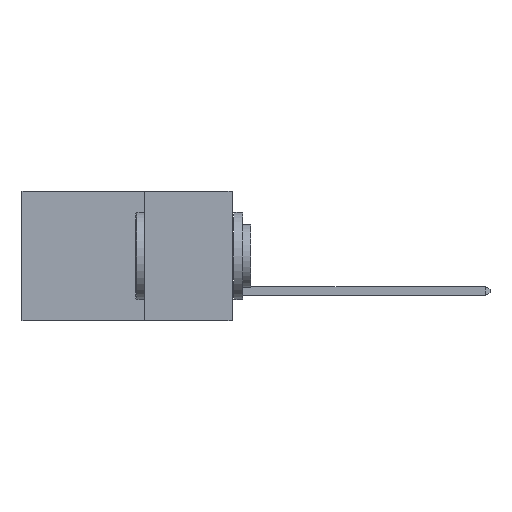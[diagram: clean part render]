
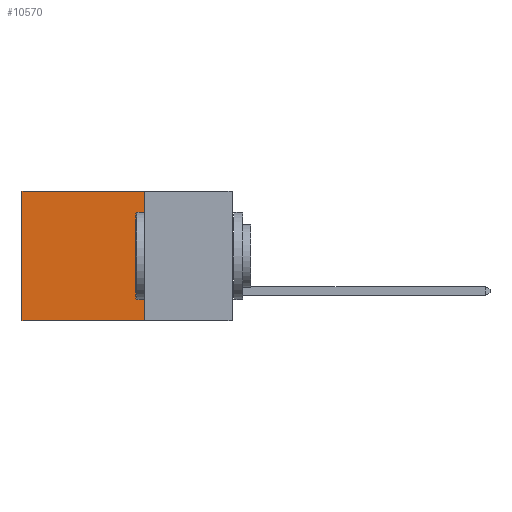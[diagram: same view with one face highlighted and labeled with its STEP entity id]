
A CAD part, left-side view. The second image highlights one B-rep face of the part: STEP entity #10570.
In plain terms, the highlighted planar face has unit normal (-1, 0, 0).
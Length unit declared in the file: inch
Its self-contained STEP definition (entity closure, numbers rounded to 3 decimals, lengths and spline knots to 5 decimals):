
#978 = VECTOR ( 'NONE', #19022, 39.37008 ) ;
#990 = VERTEX_POINT ( 'NONE', #17143 ) ;
#3026 = VECTOR ( 'NONE', #17542, 39.37008 ) ;
#3767 = DIRECTION ( 'NONE',  ( 1., 0., 0. ) ) ;
#4376 = LINE ( 'NONE', #12175, #12328 ) ;
#5429 = VERTEX_POINT ( 'NONE', #9429 ) ;
#5450 = LINE ( 'NONE', #17532, #978 ) ;
#7081 = VERTEX_POINT ( 'NONE', #13570 ) ;
#7306 = LINE ( 'NONE', #10642, #11495 ) ;
#7717 = VERTEX_POINT ( 'NONE', #15780 ) ;
#7954 = FACE_OUTER_BOUND ( 'NONE', #17458, .T. ) ;
#9429 = CARTESIAN_POINT ( 'NONE',  ( 0.2875, 0.6, 0. ) ) ;
#10570 = ADVANCED_FACE ( 'NONE', ( #7954 ), #13247, .F. ) ;
#10642 = CARTESIAN_POINT ( 'NONE',  ( 0.2875, 0.6, 0. ) ) ;
#10745 = EDGE_CURVE ( 'NONE', #990, #7081, #4376, .T. ) ;
#11495 = VECTOR ( 'NONE', #12145, 39.37008 ) ;
#12145 = DIRECTION ( 'NONE',  ( 0., 0., -1. ) ) ;
#12175 = CARTESIAN_POINT ( 'NONE',  ( 0.2875, 0.25, -0.37 ) ) ;
#12304 = AXIS2_PLACEMENT_3D ( 'NONE', #19139, #3767, #14733 ) ;
#12328 = VECTOR ( 'NONE', #13682, 39.37008 ) ;
#13247 = PLANE ( 'NONE',  #12304 ) ;
#13538 = EDGE_CURVE ( 'NONE', #5429, #7081, #7306, .T. ) ;
#13570 = CARTESIAN_POINT ( 'NONE',  ( 0.2875, 0.6, -0.37 ) ) ;
#13682 = DIRECTION ( 'NONE',  ( 0., 1., 0. ) ) ;
#14096 = ORIENTED_EDGE ( 'NONE', *, *, #17262, .T. ) ;
#14733 = DIRECTION ( 'NONE',  ( 0., 0., -1. ) ) ;
#15532 = ORIENTED_EDGE ( 'NONE', *, *, #13538, .T. ) ;
#15565 = LINE ( 'NONE', #16065, #3026 ) ;
#15709 = EDGE_CURVE ( 'NONE', #7717, #990, #5450, .T. ) ;
#15780 = CARTESIAN_POINT ( 'NONE',  ( 0.2875, 0.25, 0. ) ) ;
#16065 = CARTESIAN_POINT ( 'NONE',  ( 0.2875, 0.25, 0. ) ) ;
#17143 = CARTESIAN_POINT ( 'NONE',  ( 0.2875, 0.25, -0.37 ) ) ;
#17262 = EDGE_CURVE ( 'NONE', #7717, #5429, #15565, .T. ) ;
#17343 = ORIENTED_EDGE ( 'NONE', *, *, #15709, .F. ) ;
#17458 = EDGE_LOOP ( 'NONE', ( #15532, #20259, #17343, #14096 ) ) ;
#17532 = CARTESIAN_POINT ( 'NONE',  ( 0.2875, 0.25, 0. ) ) ;
#17542 = DIRECTION ( 'NONE',  ( 0., 1., 0. ) ) ;
#19022 = DIRECTION ( 'NONE',  ( 0., 0., -1. ) ) ;
#19139 = CARTESIAN_POINT ( 'NONE',  ( 0.2875, 0.25, 0. ) ) ;
#20259 = ORIENTED_EDGE ( 'NONE', *, *, #10745, .F. ) ;
